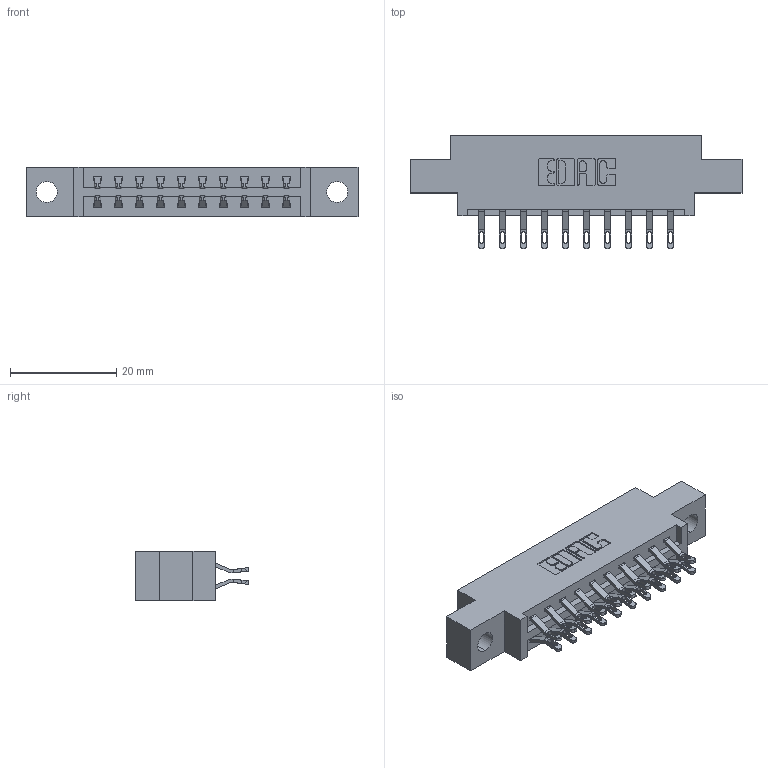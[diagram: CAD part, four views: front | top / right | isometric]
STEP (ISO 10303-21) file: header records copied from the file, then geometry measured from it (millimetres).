
FILE_DESCRIPTION (( 'STEP AP203' ), '1' );
FILE_NAME ('337-020-555-804.STEP', '2018-08-05T10:05:04', ( '' ), ( '' ), 'SwSTEP 2.0', 'SolidWorks 2016', '' );
FILE_SCHEMA (( 'CONFIG_CONTROL_DESIGN' ));
Length unit declared in the file: inch
Products named in the file (3): 337 Part_0.170 Offset - 0.156 Dia-TH; 345-292-001_555 Tail; 337-020-555-804
Assembly tree (21 placements, depth 2):
  337-020-555-804
    337 Part_0.170 Offset - 0.156 Dia-TH
    345-292-001_555 Tail  x20
Bounding box: 62.64 x 21.47 x 9.4 mm (x, y, z)
Volume: 6027.8 mm3; surface area: 6627.5 mm2
Topology: 21 solids, 21 shells, 1318 faces, 4103 edges, 2734 vertices
Faces by surface type: plane 794, cylinder 524
Entity records: 12353 total; most frequent: CARTESIAN_POINT 2144, ORIENTED_EDGE 2050, DIRECTION 1853, EDGE_CURVE 1025, LINE 877, VECTOR 877, VERTEX_POINT 682, AXIS2_PLACEMENT_3D 488
